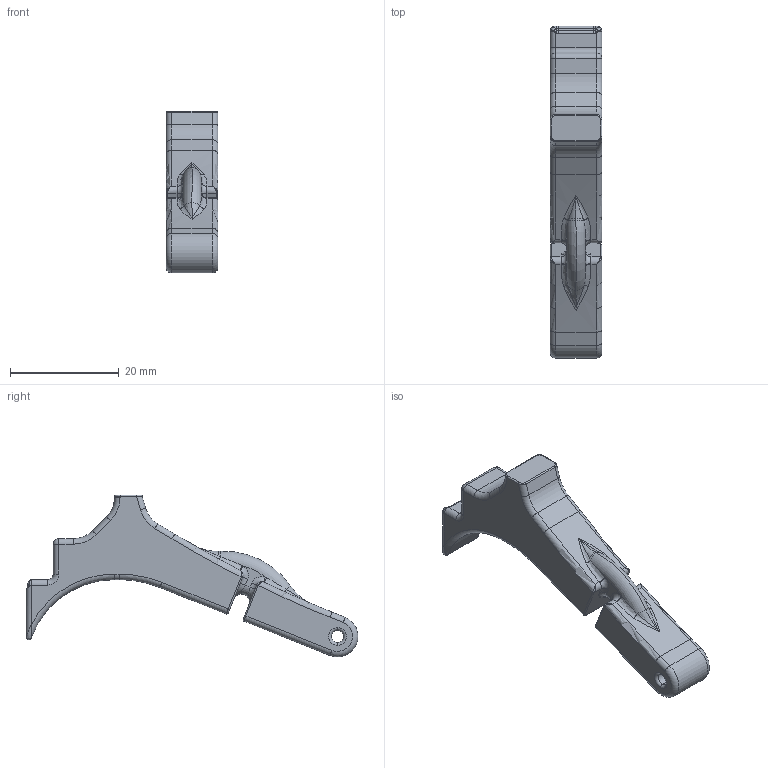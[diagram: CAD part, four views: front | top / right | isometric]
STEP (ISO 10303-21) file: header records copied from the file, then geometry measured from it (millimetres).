
FILE_DESCRIPTION (( 'STEP AP214' ), '1' );
FILE_NAME ('Hammer.STEP', '2013-11-21T02:43:07', ( '' ), ( '' ), 'SwSTEP 2.0', 'SolidWorks 2013', '' );
FILE_SCHEMA (( 'AUTOMOTIVE_DESIGN' ));
Length unit declared in the file: millimetre
Products named in the file (1): Hammer
Bounding box: 9.5 x 60.92 x 29.69 mm (x, y, z)
Volume: 5443.9 mm3; surface area: 2789.1 mm2
Topology: 1 solids, 1 shells, 226 faces, 542 edges, 286 vertices
Faces by surface type: cylinder 77, torus 64, bspline 32, plane 29, sphere 24
Entity records: 7456 total; most frequent: CARTESIAN_POINT 2475, DIRECTION 1118, ORIENTED_EDGE 1020, EDGE_CURVE 510, AXIS2_PLACEMENT_3D 491, CIRCLE 296, VERTEX_POINT 286, EDGE_LOOP 228
